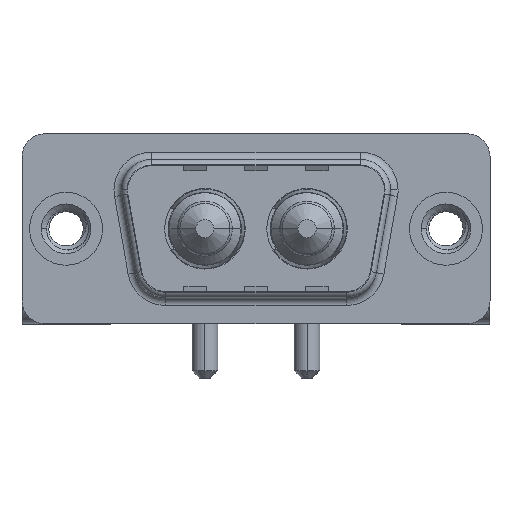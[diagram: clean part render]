
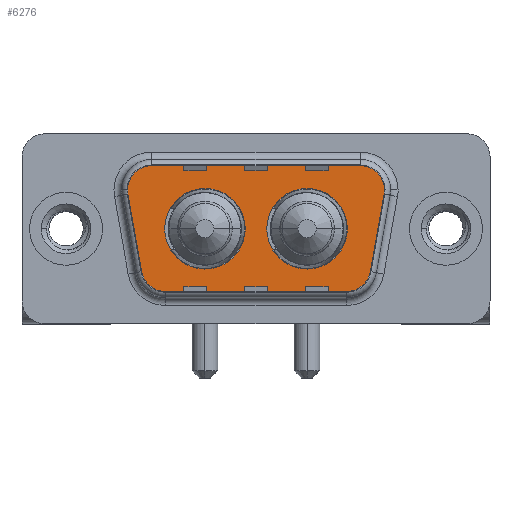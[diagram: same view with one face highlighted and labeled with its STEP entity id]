
A CAD part, top view. The second image highlights one B-rep face of the part: STEP entity #6276.
In plain terms, the highlighted planar face has unit normal (0, 0, 1).
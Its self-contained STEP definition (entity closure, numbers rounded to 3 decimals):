
#42 = DIRECTION ( 'NONE',  ( 0., 0., 1. ) ) ;
#69 = ORIENTED_EDGE ( 'NONE', *, *, #5800, .T. ) ;
#109 = DIRECTION ( 'NONE',  ( -1., 0., 0. ) ) ;
#323 = CARTESIAN_POINT ( 'NONE',  ( 5.436, 4.9, 0. ) ) ;
#402 = DIRECTION ( 'NONE',  ( 0., 0., 1. ) ) ;
#504 = EDGE_CURVE ( 'NONE', #1270, #7765, #5439, .T. ) ;
#604 = DIRECTION ( 'NONE',  ( -1., 0., 0. ) ) ;
#660 = AXIS2_PLACEMENT_3D ( 'NONE', #6026, #6956, #9803 ) ;
#811 = DIRECTION ( 'NONE',  ( 0., 0., 1. ) ) ;
#909 = CIRCLE ( 'NONE', #4882, 2. ) ;
#928 = VERTEX_POINT ( 'NONE', #6913 ) ;
#1096 = CARTESIAN_POINT ( 'NONE',  ( 21.564, 2.9, 0. ) ) ;
#1270 = VERTEX_POINT ( 'NONE', #1096 ) ;
#1328 = VERTEX_POINT ( 'NONE', #8739 ) ;
#1367 = CARTESIAN_POINT ( 'NONE',  ( 18.51, 0., 0. ) ) ;
#1537 = CARTESIAN_POINT ( 'NONE',  ( 21.534, 2.553, 0. ) ) ;
#1549 = DIRECTION ( 'NONE',  ( 0., 0., 1. ) ) ;
#1624 = CARTESIAN_POINT ( 'NONE',  ( 15.86, 0., 0. ) ) ;
#1645 = EDGE_CURVE ( 'NONE', #10360, #5415, #909, .T. ) ;
#1766 = DIRECTION ( 'NONE',  ( 0., 0., 1. ) ) ;
#1800 = DIRECTION ( 'NONE',  ( 0., 0., 1. ) ) ;
#1847 = EDGE_CURVE ( 'NONE', #11853, #12186, #7666, .T. ) ;
#1865 = ORIENTED_EDGE ( 'NONE', *, *, #1645, .T. ) ;
#1950 = VERTEX_POINT ( 'NONE', #10967 ) ;
#2031 = ORIENTED_EDGE ( 'NONE', *, *, #504, .T. ) ;
#2399 = DIRECTION ( 'NONE',  ( 1., 0., 0. ) ) ;
#2718 = CARTESIAN_POINT ( 'NONE',  ( 11.79, 0., 0. ) ) ;
#2924 = CARTESIAN_POINT ( 'NONE',  ( 9.14, 0., 0. ) ) ;
#2950 = DIRECTION ( 'NONE',  ( 0., 0., 1. ) ) ;
#3004 = ORIENTED_EDGE ( 'NONE', *, *, #4015, .F. ) ;
#3094 = DIRECTION ( 'NONE',  ( 0.174, -0.985, 0. ) ) ;
#3178 = ORIENTED_EDGE ( 'NONE', *, *, #5755, .T. ) ;
#3214 = CARTESIAN_POINT ( 'NONE',  ( 3.466, 2.553, 0. ) ) ;
#3276 = VERTEX_POINT ( 'NONE', #6247 ) ;
#3320 = DIRECTION ( 'NONE',  ( 0., 0., 1. ) ) ;
#3568 = EDGE_LOOP ( 'NONE', ( #9670, #12097 ) ) ;
#3887 = DIRECTION ( 'NONE',  ( 0., 0., 1. ) ) ;
#3916 = ORIENTED_EDGE ( 'NONE', *, *, #12200, .T. ) ;
#3921 = AXIS2_PLACEMENT_3D ( 'NONE', #11161, #1766, #7293 ) ;
#3926 = ORIENTED_EDGE ( 'NONE', *, *, #1847, .F. ) ;
#3930 = VERTEX_POINT ( 'NONE', #12079 ) ;
#3938 = AXIS2_PLACEMENT_3D ( 'NONE', #4810, #3887, #9778 ) ;
#4008 = CARTESIAN_POINT ( 'NONE',  ( 18.541, -2.9, 0. ) ) ;
#4015 = EDGE_CURVE ( 'NONE', #12186, #11853, #9779, .T. ) ;
#4063 = AXIS2_PLACEMENT_3D ( 'NONE', #11944, #1549, #604 ) ;
#4395 = LINE ( 'NONE', #1537, #11001 ) ;
#4717 = CIRCLE ( 'NONE', #5311, 2.65 ) ;
#4723 = EDGE_CURVE ( 'NONE', #3930, #928, #5710, .T. ) ;
#4810 = CARTESIAN_POINT ( 'NONE',  ( 15.86, 0., 0. ) ) ;
#4882 = AXIS2_PLACEMENT_3D ( 'NONE', #4008, #2950, #7735 ) ;
#4980 = EDGE_CURVE ( 'NONE', #1950, #1270, #11242, .T. ) ;
#5013 = CARTESIAN_POINT ( 'NONE',  ( 6.49, 0., 0. ) ) ;
#5046 = EDGE_CURVE ( 'NONE', #928, #6895, #10060, .T. ) ;
#5311 = AXIS2_PLACEMENT_3D ( 'NONE', #1624, #811, #10212 ) ;
#5375 = EDGE_LOOP ( 'NONE', ( #1865, #3178, #6014, #2031, #5799, #69, #8345, #8538, #3916 ) ) ;
#5379 = EDGE_CURVE ( 'NONE', #7765, #1328, #9070, .T. ) ;
#5415 = VERTEX_POINT ( 'NONE', #7147 ) ;
#5439 = CIRCLE ( 'NONE', #4063, 2. ) ;
#5710 = LINE ( 'NONE', #3214, #10609 ) ;
#5755 = EDGE_CURVE ( 'NONE', #5415, #1950, #4395, .T. ) ;
#5799 = ORIENTED_EDGE ( 'NONE', *, *, #5379, .T. ) ;
#5800 = EDGE_CURVE ( 'NONE', #1328, #3930, #10405, .T. ) ;
#6014 = ORIENTED_EDGE ( 'NONE', *, *, #4980, .T. ) ;
#6026 = CARTESIAN_POINT ( 'NONE',  ( 5.436, 2.9, 0. ) ) ;
#6194 = CARTESIAN_POINT ( 'NONE',  ( 18.541, -2.9, 0. ) ) ;
#6247 = CARTESIAN_POINT ( 'NONE',  ( 13.21, 0., 0. ) ) ;
#6256 = FACE_BOUND ( 'NONE', #3568, .T. ) ;
#6269 = DIRECTION ( 'NONE',  ( 0.174, 0.985, 0. ) ) ;
#6276 = ADVANCED_FACE ( 'NONE', ( #6256, #11789, #7866 ), #11922, .T. ) ;
#6895 = VERTEX_POINT ( 'NONE', #10203 ) ;
#6913 = CARTESIAN_POINT ( 'NONE',  ( 4.489, -3.247, 0. ) ) ;
#6956 = DIRECTION ( 'NONE',  ( 0., 0., 1. ) ) ;
#7059 = LINE ( 'NONE', #9978, #10319 ) ;
#7099 = EDGE_LOOP ( 'NONE', ( #3926, #3004 ) ) ;
#7105 = CARTESIAN_POINT ( 'NONE',  ( 9.14, 0., 0. ) ) ;
#7147 = CARTESIAN_POINT ( 'NONE',  ( 20.511, -3.247, 0. ) ) ;
#7293 = DIRECTION ( 'NONE',  ( -1., 0., 0. ) ) ;
#7637 = CARTESIAN_POINT ( 'NONE',  ( 19.564, 2.9, 0. ) ) ;
#7666 = CIRCLE ( 'NONE', #12049, 2.65 ) ;
#7735 = DIRECTION ( 'NONE',  ( 1., 0., 0. ) ) ;
#7765 = VERTEX_POINT ( 'NONE', #8547 ) ;
#7866 = FACE_OUTER_BOUND ( 'NONE', #5375, .T. ) ;
#8214 = CARTESIAN_POINT ( 'NONE',  ( 18.541, -4.9, 0. ) ) ;
#8345 = ORIENTED_EDGE ( 'NONE', *, *, #4723, .T. ) ;
#8538 = ORIENTED_EDGE ( 'NONE', *, *, #5046, .T. ) ;
#8547 = CARTESIAN_POINT ( 'NONE',  ( 19.564, 4.9, 0. ) ) ;
#8739 = CARTESIAN_POINT ( 'NONE',  ( 5.436, 4.9, 0. ) ) ;
#8855 = DIRECTION ( 'NONE',  ( 1., 0., 0. ) ) ;
#9070 = LINE ( 'NONE', #323, #10733 ) ;
#9169 = AXIS2_PLACEMENT_3D ( 'NONE', #2924, #42, #11383 ) ;
#9243 = AXIS2_PLACEMENT_3D ( 'NONE', #7637, #1800, #109 ) ;
#9670 = ORIENTED_EDGE ( 'NONE', *, *, #10171, .F. ) ;
#9778 = DIRECTION ( 'NONE',  ( 1., 0., 0. ) ) ;
#9779 = CIRCLE ( 'NONE', #9169, 2.65 ) ;
#9803 = DIRECTION ( 'NONE',  ( 1., 0., 0. ) ) ;
#9978 = CARTESIAN_POINT ( 'NONE',  ( 6.459, -4.9, 0. ) ) ;
#10060 = CIRCLE ( 'NONE', #3921, 2. ) ;
#10171 = EDGE_CURVE ( 'NONE', #11265, #3276, #11084, .T. ) ;
#10203 = CARTESIAN_POINT ( 'NONE',  ( 6.459, -4.9, 0. ) ) ;
#10212 = DIRECTION ( 'NONE',  ( 1., 0., 0. ) ) ;
#10319 = VECTOR ( 'NONE', #2399, 1000. ) ;
#10360 = VERTEX_POINT ( 'NONE', #8214 ) ;
#10372 = EDGE_CURVE ( 'NONE', #3276, #11265, #4717, .T. ) ;
#10405 = CIRCLE ( 'NONE', #660, 2. ) ;
#10609 = VECTOR ( 'NONE', #3094, 1000. ) ;
#10651 = AXIS2_PLACEMENT_3D ( 'NONE', #6194, #402, #8855 ) ;
#10733 = VECTOR ( 'NONE', #11012, 1000. ) ;
#10910 = DIRECTION ( 'NONE',  ( 1., 0., 0. ) ) ;
#10967 = CARTESIAN_POINT ( 'NONE',  ( 21.534, 2.553, 0. ) ) ;
#11001 = VECTOR ( 'NONE', #6269, 1000. ) ;
#11012 = DIRECTION ( 'NONE',  ( -1., 0., 0. ) ) ;
#11084 = CIRCLE ( 'NONE', #3938, 2.65 ) ;
#11161 = CARTESIAN_POINT ( 'NONE',  ( 6.459, -2.9, 0. ) ) ;
#11242 = CIRCLE ( 'NONE', #9243, 2. ) ;
#11265 = VERTEX_POINT ( 'NONE', #1367 ) ;
#11383 = DIRECTION ( 'NONE',  ( 1., 0., 0. ) ) ;
#11789 = FACE_BOUND ( 'NONE', #7099, .T. ) ;
#11853 = VERTEX_POINT ( 'NONE', #2718 ) ;
#11922 = PLANE ( 'NONE',  #10651 ) ;
#11944 = CARTESIAN_POINT ( 'NONE',  ( 19.564, 2.9, 0. ) ) ;
#12049 = AXIS2_PLACEMENT_3D ( 'NONE', #7105, #3320, #10910 ) ;
#12079 = CARTESIAN_POINT ( 'NONE',  ( 3.466, 2.553, 0. ) ) ;
#12097 = ORIENTED_EDGE ( 'NONE', *, *, #10372, .F. ) ;
#12186 = VERTEX_POINT ( 'NONE', #5013 ) ;
#12200 = EDGE_CURVE ( 'NONE', #6895, #10360, #7059, .T. ) ;
